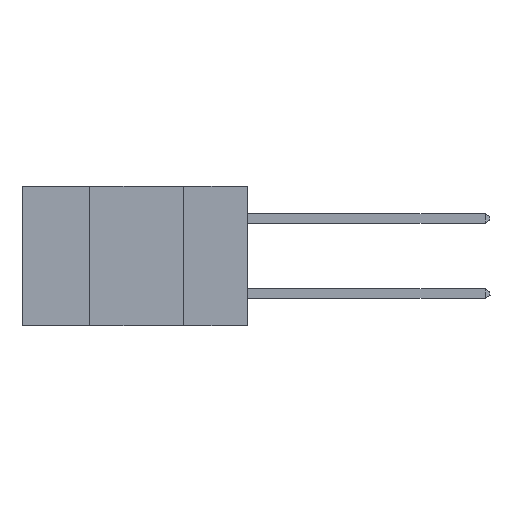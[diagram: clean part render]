
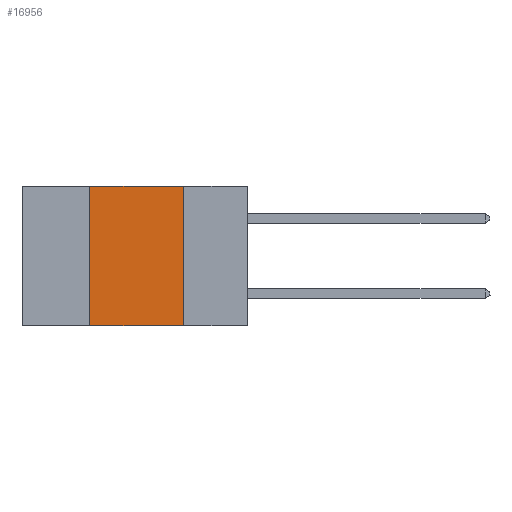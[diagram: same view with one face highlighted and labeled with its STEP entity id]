
A CAD part, left-side view. The second image highlights one B-rep face of the part: STEP entity #16956.
In plain terms, the highlighted planar face has unit normal (-1, 0, 0).
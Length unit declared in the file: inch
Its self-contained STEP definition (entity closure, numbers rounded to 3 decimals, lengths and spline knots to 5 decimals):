
#240 = DIRECTION ( 'NONE',  ( 0., 0., -1. ) ) ;
#672 = VECTOR ( 'NONE', #240, 39.37008 ) ;
#723 = VECTOR ( 'NONE', #13827, 39.37008 ) ;
#1003 = EDGE_LOOP ( 'NONE', ( #4365, #1355, #5917, #12299 ) ) ;
#1355 = ORIENTED_EDGE ( 'NONE', *, *, #3611, .F. ) ;
#1702 = VERTEX_POINT ( 'NONE', #3859 ) ;
#2295 = VERTEX_POINT ( 'NONE', #10845 ) ;
#2407 = CARTESIAN_POINT ( 'NONE',  ( 0., 0.42, 0. ) ) ;
#3611 = EDGE_CURVE ( 'NONE', #11850, #7874, #13840, .T. ) ;
#3859 = CARTESIAN_POINT ( 'NONE',  ( 0., 0.42, -0.37 ) ) ;
#4365 = ORIENTED_EDGE ( 'NONE', *, *, #17109, .F. ) ;
#4529 = CARTESIAN_POINT ( 'NONE',  ( 0., 0.6, 0. ) ) ;
#4718 = PLANE ( 'NONE',  #5953 ) ;
#4899 = DIRECTION ( 'NONE',  ( 1., 0., 0. ) ) ;
#5390 = CARTESIAN_POINT ( 'NONE',  ( 0., 0.42, 0. ) ) ;
#5575 = CARTESIAN_POINT ( 'NONE',  ( 0., 0.17, 0. ) ) ;
#5917 = ORIENTED_EDGE ( 'NONE', *, *, #7268, .F. ) ;
#5953 = AXIS2_PLACEMENT_3D ( 'NONE', #15214, #4899, #15274 ) ;
#6353 = LINE ( 'NONE', #5390, #14187 ) ;
#7268 = EDGE_CURVE ( 'NONE', #1702, #11850, #6353, .T. ) ;
#7874 = VERTEX_POINT ( 'NONE', #9787 ) ;
#7962 = EDGE_CURVE ( 'NONE', #1702, #2295, #9421, .T. ) ;
#9421 = LINE ( 'NONE', #12473, #14357 ) ;
#9614 = DIRECTION ( 'NONE',  ( 0., 0., 1. ) ) ;
#9787 = CARTESIAN_POINT ( 'NONE',  ( 0., 0.17, 0. ) ) ;
#10845 = CARTESIAN_POINT ( 'NONE',  ( 0., 0.17, -0.37 ) ) ;
#11233 = DIRECTION ( 'NONE',  ( 0., -1., 0. ) ) ;
#11310 = LINE ( 'NONE', #5575, #672 ) ;
#11850 = VERTEX_POINT ( 'NONE', #2407 ) ;
#12299 = ORIENTED_EDGE ( 'NONE', *, *, #7962, .T. ) ;
#12473 = CARTESIAN_POINT ( 'NONE',  ( 0., 0.6, -0.37 ) ) ;
#13151 = FACE_OUTER_BOUND ( 'NONE', #1003, .T. ) ;
#13827 = DIRECTION ( 'NONE',  ( 0., -1., 0. ) ) ;
#13840 = LINE ( 'NONE', #4529, #723 ) ;
#14187 = VECTOR ( 'NONE', #9614, 39.37008 ) ;
#14357 = VECTOR ( 'NONE', #11233, 39.37008 ) ;
#15214 = CARTESIAN_POINT ( 'NONE',  ( 0., 0.6, 0. ) ) ;
#15274 = DIRECTION ( 'NONE',  ( 0., 0., -1. ) ) ;
#16956 = ADVANCED_FACE ( 'NONE', ( #13151 ), #4718, .F. ) ;
#17109 = EDGE_CURVE ( 'NONE', #7874, #2295, #11310, .T. ) ;
